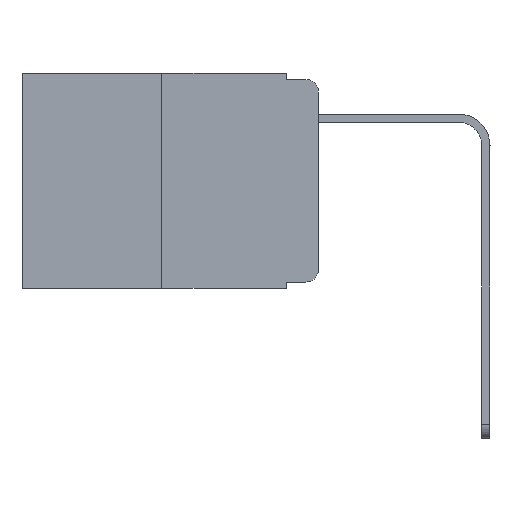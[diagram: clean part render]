
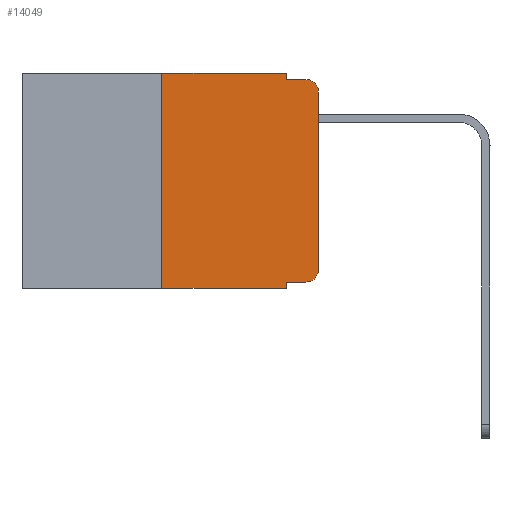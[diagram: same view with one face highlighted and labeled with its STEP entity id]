
A CAD part, left-side view. The second image highlights one B-rep face of the part: STEP entity #14049.
In plain terms, the highlighted planar face has unit normal (-1, 0, 0).
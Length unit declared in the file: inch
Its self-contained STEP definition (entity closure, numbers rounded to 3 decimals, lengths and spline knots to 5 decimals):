
#202 = ORIENTED_EDGE ( 'NONE', *, *, #3052, .T. ) ;
#561 = VECTOR ( 'NONE', #14198, 39.37008 ) ;
#731 = CARTESIAN_POINT ( 'NONE',  ( 0., 0.051, -0.333 ) ) ;
#813 = EDGE_CURVE ( 'NONE', #1454, #11653, #3580, .T. ) ;
#1011 = LINE ( 'NONE', #7035, #10666 ) ;
#1454 = VERTEX_POINT ( 'NONE', #3516 ) ;
#1514 = ORIENTED_EDGE ( 'NONE', *, *, #13704, .T. ) ;
#1651 = CARTESIAN_POINT ( 'NONE',  ( 0., 0.02, -0.03 ) ) ;
#2136 = FACE_OUTER_BOUND ( 'NONE', #3431, .T. ) ;
#2230 = LINE ( 'NONE', #5986, #3805 ) ;
#2324 = CARTESIAN_POINT ( 'NONE',  ( 0., 0.473, 0. ) ) ;
#2497 = CARTESIAN_POINT ( 'NONE',  ( 0., 0., -0.313 ) ) ;
#2558 = PLANE ( 'NONE',  #6062 ) ;
#2610 = CARTESIAN_POINT ( 'NONE',  ( 0., 0.051, 0. ) ) ;
#2776 = DIRECTION ( 'NONE',  ( 0., 0., -1. ) ) ;
#2816 = ORIENTED_EDGE ( 'NONE', *, *, #14558, .F. ) ;
#3020 = LINE ( 'NONE', #731, #561 ) ;
#3052 = EDGE_CURVE ( 'NONE', #7503, #7829, #1011, .T. ) ;
#3220 = ORIENTED_EDGE ( 'NONE', *, *, #8130, .T. ) ;
#3431 = EDGE_LOOP ( 'NONE', ( #202, #10928, #7506, #12285, #4943, #2816, #3220, #8377, #1514, #6918 ) ) ;
#3516 = CARTESIAN_POINT ( 'NONE',  ( 0., 0.25, 0. ) ) ;
#3580 = LINE ( 'NONE', #2324, #9769 ) ;
#3600 = AXIS2_PLACEMENT_3D ( 'NONE', #13111, #7531, #7427 ) ;
#3805 = VECTOR ( 'NONE', #4906, 39.37008 ) ;
#3834 = DIRECTION ( 'NONE',  ( 0., -1., 0. ) ) ;
#4258 = VERTEX_POINT ( 'NONE', #10206 ) ;
#4906 = DIRECTION ( 'NONE',  ( 0., 0., -1. ) ) ;
#4917 = CARTESIAN_POINT ( 'NONE',  ( 0., 0.051, -0.01 ) ) ;
#4943 = ORIENTED_EDGE ( 'NONE', *, *, #813, .F. ) ;
#4959 = CARTESIAN_POINT ( 'NONE',  ( 0., 0.25, 0. ) ) ;
#5895 = VERTEX_POINT ( 'NONE', #7373 ) ;
#5986 = CARTESIAN_POINT ( 'NONE',  ( 0., 0.051, 0. ) ) ;
#6062 = AXIS2_PLACEMENT_3D ( 'NONE', #6221, #10418, #9203 ) ;
#6221 = CARTESIAN_POINT ( 'NONE',  ( 0., 0.473, 0. ) ) ;
#6233 = VECTOR ( 'NONE', #12777, 39.37008 ) ;
#6770 = CARTESIAN_POINT ( 'NONE',  ( 0., 0., -0.03 ) ) ;
#6861 = EDGE_CURVE ( 'NONE', #7829, #7202, #10609, .T. ) ;
#6862 = AXIS2_PLACEMENT_3D ( 'NONE', #1651, #9531, #2776 ) ;
#6918 = ORIENTED_EDGE ( 'NONE', *, *, #13725, .T. ) ;
#7035 = CARTESIAN_POINT ( 'NONE',  ( 0., 0., 0. ) ) ;
#7079 = DIRECTION ( 'NONE',  ( 0., 0., 1. ) ) ;
#7097 = DIRECTION ( 'NONE',  ( 0., 0., 1. ) ) ;
#7202 = VERTEX_POINT ( 'NONE', #13651 ) ;
#7373 = CARTESIAN_POINT ( 'NONE',  ( 0., 0.051, -0.343 ) ) ;
#7427 = DIRECTION ( 'NONE',  ( 0., 0., -1. ) ) ;
#7489 = VECTOR ( 'NONE', #13734, 39.37008 ) ;
#7503 = VERTEX_POINT ( 'NONE', #2497 ) ;
#7506 = ORIENTED_EDGE ( 'NONE', *, *, #14561, .F. ) ;
#7531 = DIRECTION ( 'NONE',  ( -1., 0., 0. ) ) ;
#7636 = VERTEX_POINT ( 'NONE', #13095 ) ;
#7829 = VERTEX_POINT ( 'NONE', #6770 ) ;
#8130 = EDGE_CURVE ( 'NONE', #4258, #5895, #8526, .T. ) ;
#8341 = CARTESIAN_POINT ( 'NONE',  ( 0., 0.051, -0.01 ) ) ;
#8377 = ORIENTED_EDGE ( 'NONE', *, *, #11395, .F. ) ;
#8460 = VECTOR ( 'NONE', #7097, 39.37008 ) ;
#8526 = LINE ( 'NONE', #11644, #6233 ) ;
#8670 = CIRCLE ( 'NONE', #3600, 0.02 ) ;
#9203 = DIRECTION ( 'NONE',  ( 0., 0., -1. ) ) ;
#9531 = DIRECTION ( 'NONE',  ( -1., 0., 0. ) ) ;
#9769 = VECTOR ( 'NONE', #10334, 39.37008 ) ;
#9864 = LINE ( 'NONE', #4917, #14427 ) ;
#10011 = EDGE_CURVE ( 'NONE', #11653, #10245, #2230, .T. ) ;
#10206 = CARTESIAN_POINT ( 'NONE',  ( 0., 0.25, -0.343 ) ) ;
#10245 = VERTEX_POINT ( 'NONE', #8341 ) ;
#10334 = DIRECTION ( 'NONE',  ( 0., -1., 0. ) ) ;
#10418 = DIRECTION ( 'NONE',  ( 1., 0., 0. ) ) ;
#10608 = LINE ( 'NONE', #2610, #7489 ) ;
#10609 = CIRCLE ( 'NONE', #6862, 0.02 ) ;
#10666 = VECTOR ( 'NONE', #7079, 39.37008 ) ;
#10928 = ORIENTED_EDGE ( 'NONE', *, *, #6861, .T. ) ;
#11395 = EDGE_CURVE ( 'NONE', #7636, #5895, #10608, .T. ) ;
#11578 = CARTESIAN_POINT ( 'NONE',  ( 0., 0.02, -0.333 ) ) ;
#11644 = CARTESIAN_POINT ( 'NONE',  ( 0., 0.473, -0.343 ) ) ;
#11653 = VERTEX_POINT ( 'NONE', #14373 ) ;
#12285 = ORIENTED_EDGE ( 'NONE', *, *, #10011, .F. ) ;
#12777 = DIRECTION ( 'NONE',  ( 0., -1., 0. ) ) ;
#13095 = CARTESIAN_POINT ( 'NONE',  ( 0., 0.051, -0.333 ) ) ;
#13111 = CARTESIAN_POINT ( 'NONE',  ( 0., 0.02, -0.313 ) ) ;
#13461 = VERTEX_POINT ( 'NONE', #11578 ) ;
#13651 = CARTESIAN_POINT ( 'NONE',  ( 0., 0.02, -0.01 ) ) ;
#13704 = EDGE_CURVE ( 'NONE', #7636, #13461, #3020, .T. ) ;
#13725 = EDGE_CURVE ( 'NONE', #13461, #7503, #8670, .T. ) ;
#13734 = DIRECTION ( 'NONE',  ( 0., 0., -1. ) ) ;
#14049 = ADVANCED_FACE ( 'NONE', ( #2136 ), #2558, .F. ) ;
#14083 = LINE ( 'NONE', #4959, #8460 ) ;
#14198 = DIRECTION ( 'NONE',  ( 0., -1., 0. ) ) ;
#14373 = CARTESIAN_POINT ( 'NONE',  ( 0., 0.051, 0. ) ) ;
#14427 = VECTOR ( 'NONE', #3834, 39.37008 ) ;
#14558 = EDGE_CURVE ( 'NONE', #4258, #1454, #14083, .T. ) ;
#14561 = EDGE_CURVE ( 'NONE', #10245, #7202, #9864, .T. ) ;
